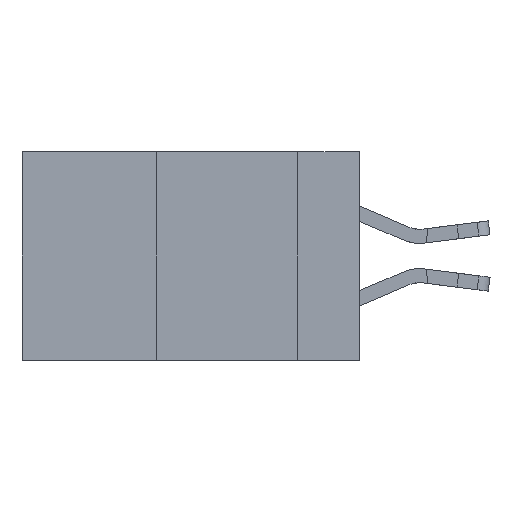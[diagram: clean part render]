
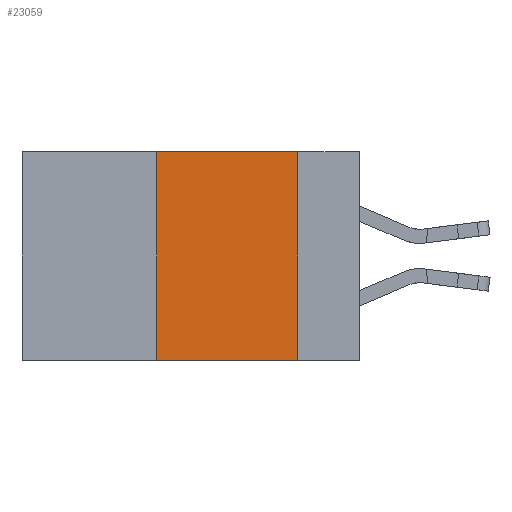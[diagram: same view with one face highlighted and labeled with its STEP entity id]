
A CAD part, left-side view. The second image highlights one B-rep face of the part: STEP entity #23059.
In plain terms, the highlighted planar face has unit normal (-1, 0, 0).
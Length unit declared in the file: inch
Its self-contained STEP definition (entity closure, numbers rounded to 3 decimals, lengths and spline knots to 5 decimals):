
#99 = VERTEX_POINT ( 'NONE', #24426 ) ;
#174 = AXIS2_PLACEMENT_3D ( 'NONE', #1670, #16715, #3829 ) ;
#1277 = CARTESIAN_POINT ( 'NONE',  ( 0., 0.6, 0. ) ) ;
#1520 = ORIENTED_EDGE ( 'NONE', *, *, #7288, .F. ) ;
#1670 = CARTESIAN_POINT ( 'NONE',  ( 0., 0.6, 0. ) ) ;
#2911 = EDGE_CURVE ( 'NONE', #20176, #12586, #3833, .T. ) ;
#3074 = VECTOR ( 'NONE', #7685, 39.37008 ) ;
#3829 = DIRECTION ( 'NONE',  ( 0., 0., -1. ) ) ;
#3833 = LINE ( 'NONE', #16816, #25871 ) ;
#4330 = EDGE_CURVE ( 'NONE', #8442, #12586, #20195, .T. ) ;
#7288 = EDGE_CURVE ( 'NONE', #8442, #99, #26963, .T. ) ;
#7685 = DIRECTION ( 'NONE',  ( 0., -1., 0. ) ) ;
#8442 = VERTEX_POINT ( 'NONE', #17578 ) ;
#8642 = FACE_OUTER_BOUND ( 'NONE', #17752, .T. ) ;
#8707 = VECTOR ( 'NONE', #8970, 39.37008 ) ;
#8970 = DIRECTION ( 'NONE',  ( 0., 0., 1. ) ) ;
#12490 = PLANE ( 'NONE',  #174 ) ;
#12586 = VERTEX_POINT ( 'NONE', #18402 ) ;
#14196 = DIRECTION ( 'NONE',  ( 0., -1., 0. ) ) ;
#15966 = ORIENTED_EDGE ( 'NONE', *, *, #2911, .F. ) ;
#16013 = CARTESIAN_POINT ( 'NONE',  ( 0., 0.6, -0.37 ) ) ;
#16715 = DIRECTION ( 'NONE',  ( 1., 0., 0. ) ) ;
#16816 = CARTESIAN_POINT ( 'NONE',  ( 0., 0.11, 0. ) ) ;
#17578 = CARTESIAN_POINT ( 'NONE',  ( 0., 0.36, -0.37 ) ) ;
#17752 = EDGE_LOOP ( 'NONE', ( #15966, #25573, #1520, #24266 ) ) ;
#18402 = CARTESIAN_POINT ( 'NONE',  ( 0., 0.11, -0.37 ) ) ;
#19111 = DIRECTION ( 'NONE',  ( 0., 0., -1. ) ) ;
#19574 = CARTESIAN_POINT ( 'NONE',  ( 0., 0.36, 0. ) ) ;
#20176 = VERTEX_POINT ( 'NONE', #26943 ) ;
#20195 = LINE ( 'NONE', #16013, #3074 ) ;
#20838 = EDGE_CURVE ( 'NONE', #99, #20176, #25990, .T. ) ;
#23059 = ADVANCED_FACE ( 'NONE', ( #8642 ), #12490, .F. ) ;
#24266 = ORIENTED_EDGE ( 'NONE', *, *, #4330, .T. ) ;
#24426 = CARTESIAN_POINT ( 'NONE',  ( 0., 0.36, 0. ) ) ;
#25573 = ORIENTED_EDGE ( 'NONE', *, *, #20838, .F. ) ;
#25871 = VECTOR ( 'NONE', #19111, 39.37008 ) ;
#25990 = LINE ( 'NONE', #1277, #26640 ) ;
#26640 = VECTOR ( 'NONE', #14196, 39.37008 ) ;
#26943 = CARTESIAN_POINT ( 'NONE',  ( 0., 0.11, 0. ) ) ;
#26963 = LINE ( 'NONE', #19574, #8707 ) ;
